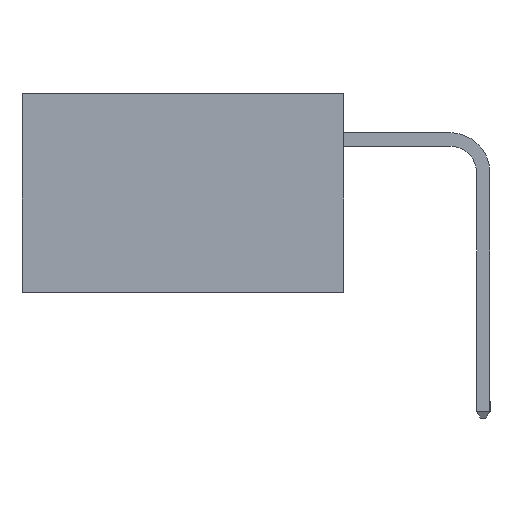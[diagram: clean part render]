
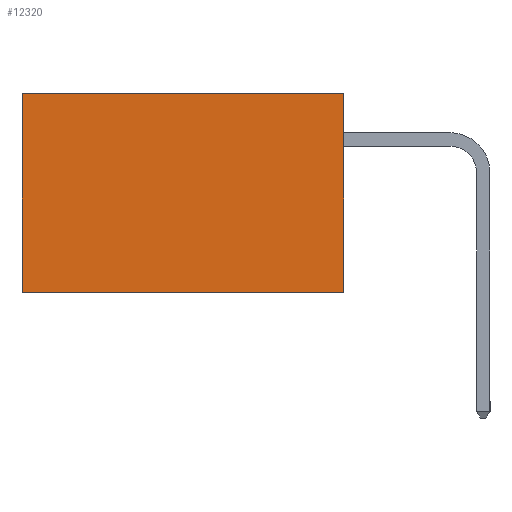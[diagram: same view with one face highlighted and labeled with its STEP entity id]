
A CAD part, left-side view. The second image highlights one B-rep face of the part: STEP entity #12320.
In plain terms, the highlighted planar face has unit normal (-1, 0, 0).
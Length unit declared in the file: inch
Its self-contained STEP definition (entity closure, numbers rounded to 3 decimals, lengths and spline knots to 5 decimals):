
#542 = EDGE_LOOP ( 'NONE', ( #9743, #14577, #13755, #7937 ) ) ;
#2037 = CARTESIAN_POINT ( 'NONE',  ( 0.2615, 0., -0.37 ) ) ;
#3466 = CARTESIAN_POINT ( 'NONE',  ( 0.2615, 0.6, -0.37 ) ) ;
#3692 = VECTOR ( 'NONE', #11183, 39.37008 ) ;
#3861 = VECTOR ( 'NONE', #6599, 39.37008 ) ;
#3977 = CARTESIAN_POINT ( 'NONE',  ( 0.2615, 0., 0. ) ) ;
#4225 = LINE ( 'NONE', #14546, #3861 ) ;
#4230 = CARTESIAN_POINT ( 'NONE',  ( 0.2615, 0., -0.37 ) ) ;
#4514 = CARTESIAN_POINT ( 'NONE',  ( 0.2615, 0., -0.37 ) ) ;
#4634 = DIRECTION ( 'NONE',  ( 0., 0., -1. ) ) ;
#4641 = VERTEX_POINT ( 'NONE', #4690 ) ;
#4675 = VERTEX_POINT ( 'NONE', #3977 ) ;
#4690 = CARTESIAN_POINT ( 'NONE',  ( 0.2615, 0.6, -0.37 ) ) ;
#5111 = AXIS2_PLACEMENT_3D ( 'NONE', #4230, #6552, #14445 ) ;
#5480 = VERTEX_POINT ( 'NONE', #4514 ) ;
#6552 = DIRECTION ( 'NONE',  ( 1., 0., 0. ) ) ;
#6599 = DIRECTION ( 'NONE',  ( 0., 0., -1. ) ) ;
#6990 = VECTOR ( 'NONE', #7072, 39.37008 ) ;
#7072 = DIRECTION ( 'NONE',  ( 0., 1., 0. ) ) ;
#7937 = ORIENTED_EDGE ( 'NONE', *, *, #11126, .T. ) ;
#8703 = LINE ( 'NONE', #3466, #14316 ) ;
#8743 = EDGE_CURVE ( 'NONE', #12995, #4641, #8703, .T. ) ;
#9167 = CARTESIAN_POINT ( 'NONE',  ( 0.2615, 0.6, 0. ) ) ;
#9743 = ORIENTED_EDGE ( 'NONE', *, *, #8743, .T. ) ;
#10006 = LINE ( 'NONE', #11556, #6990 ) ;
#11126 = EDGE_CURVE ( 'NONE', #4675, #12995, #10006, .T. ) ;
#11183 = DIRECTION ( 'NONE',  ( 0., 1., 0. ) ) ;
#11556 = CARTESIAN_POINT ( 'NONE',  ( 0.2615, 0., 0. ) ) ;
#12078 = LINE ( 'NONE', #2037, #3692 ) ;
#12320 = ADVANCED_FACE ( 'NONE', ( #12801 ), #13331, .F. ) ;
#12801 = FACE_OUTER_BOUND ( 'NONE', #542, .T. ) ;
#12866 = EDGE_CURVE ( 'NONE', #5480, #4641, #12078, .T. ) ;
#12995 = VERTEX_POINT ( 'NONE', #9167 ) ;
#13331 = PLANE ( 'NONE',  #5111 ) ;
#13755 = ORIENTED_EDGE ( 'NONE', *, *, #14213, .F. ) ;
#14213 = EDGE_CURVE ( 'NONE', #4675, #5480, #4225, .T. ) ;
#14316 = VECTOR ( 'NONE', #4634, 39.37008 ) ;
#14445 = DIRECTION ( 'NONE',  ( 0., 0., -1. ) ) ;
#14546 = CARTESIAN_POINT ( 'NONE',  ( 0.2615, 0., -0.37 ) ) ;
#14577 = ORIENTED_EDGE ( 'NONE', *, *, #12866, .F. ) ;
